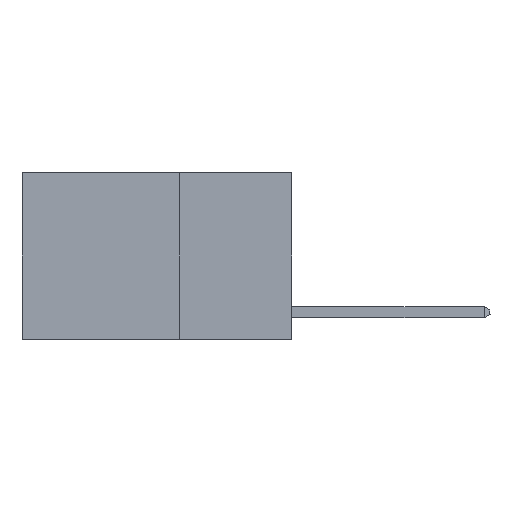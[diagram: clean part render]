
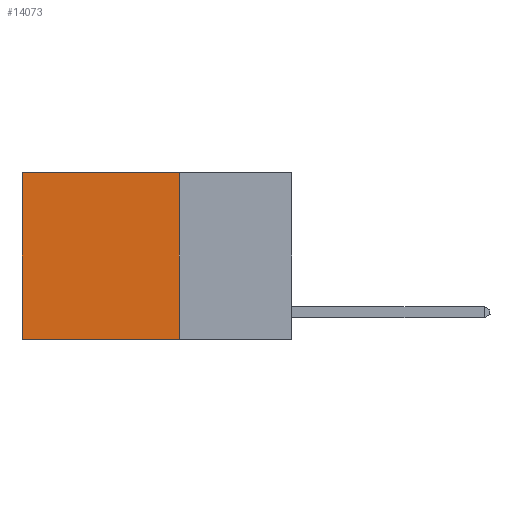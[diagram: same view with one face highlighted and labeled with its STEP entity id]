
A CAD part, left-side view. The second image highlights one B-rep face of the part: STEP entity #14073.
In plain terms, the highlighted planar face has unit normal (-1, 0, 0).
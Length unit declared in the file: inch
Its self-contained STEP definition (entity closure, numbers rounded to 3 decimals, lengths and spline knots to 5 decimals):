
#224 = VERTEX_POINT ( 'NONE', #2805 ) ;
#834 = AXIS2_PLACEMENT_3D ( 'NONE', #6996, #14281, #9630 ) ;
#1843 = VECTOR ( 'NONE', #7447, 39.37008 ) ;
#1881 = VERTEX_POINT ( 'NONE', #10055 ) ;
#2237 = ORIENTED_EDGE ( 'NONE', *, *, #8808, .F. ) ;
#2805 = CARTESIAN_POINT ( 'NONE',  ( 0.2625, 0.25, -0.37 ) ) ;
#2823 = EDGE_LOOP ( 'NONE', ( #13938, #7689, #2237, #4753 ) ) ;
#2841 = CARTESIAN_POINT ( 'NONE',  ( 0.2625, 0.6, -0.37 ) ) ;
#2911 = VERTEX_POINT ( 'NONE', #2841 ) ;
#3138 = CARTESIAN_POINT ( 'NONE',  ( 0.2625, 0.6, 0. ) ) ;
#3393 = VECTOR ( 'NONE', #3731, 39.37008 ) ;
#3731 = DIRECTION ( 'NONE',  ( 0., 1., 0. ) ) ;
#3756 = CARTESIAN_POINT ( 'NONE',  ( 0.2625, 0.25, 0. ) ) ;
#4269 = LINE ( 'NONE', #7700, #5503 ) ;
#4491 = FACE_OUTER_BOUND ( 'NONE', #2823, .T. ) ;
#4753 = ORIENTED_EDGE ( 'NONE', *, *, #8429, .T. ) ;
#5503 = VECTOR ( 'NONE', #9245, 39.37008 ) ;
#6940 = DIRECTION ( 'NONE',  ( 0., 0., -1. ) ) ;
#6996 = CARTESIAN_POINT ( 'NONE',  ( 0.2625, 0.25, 0. ) ) ;
#7278 = CARTESIAN_POINT ( 'NONE',  ( 0.2625, 0.25, 0. ) ) ;
#7447 = DIRECTION ( 'NONE',  ( 0., 0., -1. ) ) ;
#7689 = ORIENTED_EDGE ( 'NONE', *, *, #13423, .F. ) ;
#7700 = CARTESIAN_POINT ( 'NONE',  ( 0.2625, 0.25, -0.37 ) ) ;
#8429 = EDGE_CURVE ( 'NONE', #15496, #1881, #8622, .T. ) ;
#8460 = CARTESIAN_POINT ( 'NONE',  ( 0.2625, 0.25, 0. ) ) ;
#8622 = LINE ( 'NONE', #8460, #3393 ) ;
#8637 = EDGE_CURVE ( 'NONE', #1881, #2911, #15606, .T. ) ;
#8808 = EDGE_CURVE ( 'NONE', #15496, #224, #14721, .T. ) ;
#9245 = DIRECTION ( 'NONE',  ( 0., 1., 0. ) ) ;
#9630 = DIRECTION ( 'NONE',  ( 0., 0., -1. ) ) ;
#10055 = CARTESIAN_POINT ( 'NONE',  ( 0.2625, 0.6, 0. ) ) ;
#11759 = PLANE ( 'NONE',  #834 ) ;
#13423 = EDGE_CURVE ( 'NONE', #224, #2911, #4269, .T. ) ;
#13938 = ORIENTED_EDGE ( 'NONE', *, *, #8637, .T. ) ;
#14073 = ADVANCED_FACE ( 'NONE', ( #4491 ), #11759, .F. ) ;
#14281 = DIRECTION ( 'NONE',  ( 1., 0., 0. ) ) ;
#14357 = VECTOR ( 'NONE', #6940, 39.37008 ) ;
#14721 = LINE ( 'NONE', #7278, #1843 ) ;
#15496 = VERTEX_POINT ( 'NONE', #3756 ) ;
#15606 = LINE ( 'NONE', #3138, #14357 ) ;
